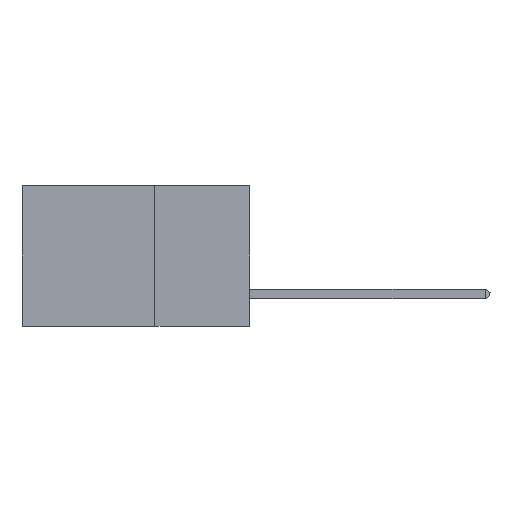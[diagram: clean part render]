
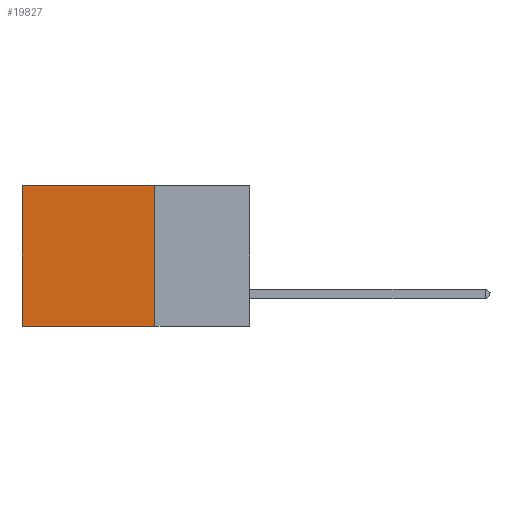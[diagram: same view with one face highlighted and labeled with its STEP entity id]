
A CAD part, left-side view. The second image highlights one B-rep face of the part: STEP entity #19827.
In plain terms, the highlighted planar face has unit normal (-1, 0, 0).
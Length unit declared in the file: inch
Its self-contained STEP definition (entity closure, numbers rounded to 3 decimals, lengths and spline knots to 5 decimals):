
#174 = EDGE_CURVE ( 'NONE', #9367, #7639, #6510, .T. ) ;
#503 = VERTEX_POINT ( 'NONE', #18927 ) ;
#1155 = ORIENTED_EDGE ( 'NONE', *, *, #21049, .F. ) ;
#1613 = CARTESIAN_POINT ( 'NONE',  ( 0.2875, 0.25, -0.37 ) ) ;
#5132 = ORIENTED_EDGE ( 'NONE', *, *, #18564, .T. ) ;
#6510 = LINE ( 'NONE', #1613, #17146 ) ;
#7128 = VECTOR ( 'NONE', #24020, 39.37008 ) ;
#7312 = DIRECTION ( 'NONE',  ( 0., 1., 0. ) ) ;
#7639 = VERTEX_POINT ( 'NONE', #15843 ) ;
#7976 = LINE ( 'NONE', #23427, #15790 ) ;
#9364 = AXIS2_PLACEMENT_3D ( 'NONE', #12331, #18625, #16492 ) ;
#9367 = VERTEX_POINT ( 'NONE', #23784 ) ;
#11425 = EDGE_LOOP ( 'NONE', ( #5132, #20590, #1155, #17836 ) ) ;
#11676 = DIRECTION ( 'NONE',  ( 0., 1., 0. ) ) ;
#11764 = EDGE_CURVE ( 'NONE', #503, #22747, #7976, .T. ) ;
#11805 = CARTESIAN_POINT ( 'NONE',  ( 0.2875, 0.25, 0. ) ) ;
#12331 = CARTESIAN_POINT ( 'NONE',  ( 0.2875, 0.25, 0. ) ) ;
#12833 = LINE ( 'NONE', #13109, #12863 ) ;
#12863 = VECTOR ( 'NONE', #19253, 39.37008 ) ;
#13109 = CARTESIAN_POINT ( 'NONE',  ( 0.2875, 0.6, 0. ) ) ;
#15790 = VECTOR ( 'NONE', #7312, 39.37008 ) ;
#15843 = CARTESIAN_POINT ( 'NONE',  ( 0.2875, 0.6, -0.37 ) ) ;
#16492 = DIRECTION ( 'NONE',  ( 0., 0., -1. ) ) ;
#17146 = VECTOR ( 'NONE', #11676, 39.37008 ) ;
#17836 = ORIENTED_EDGE ( 'NONE', *, *, #11764, .T. ) ;
#18387 = LINE ( 'NONE', #11805, #7128 ) ;
#18564 = EDGE_CURVE ( 'NONE', #22747, #7639, #12833, .T. ) ;
#18625 = DIRECTION ( 'NONE',  ( 1., 0., 0. ) ) ;
#18927 = CARTESIAN_POINT ( 'NONE',  ( 0.2875, 0.25, 0. ) ) ;
#19253 = DIRECTION ( 'NONE',  ( 0., 0., -1. ) ) ;
#19827 = ADVANCED_FACE ( 'NONE', ( #22830 ), #20473, .F. ) ;
#20473 = PLANE ( 'NONE',  #9364 ) ;
#20590 = ORIENTED_EDGE ( 'NONE', *, *, #174, .F. ) ;
#21049 = EDGE_CURVE ( 'NONE', #503, #9367, #18387, .T. ) ;
#21514 = CARTESIAN_POINT ( 'NONE',  ( 0.2875, 0.6, 0. ) ) ;
#22747 = VERTEX_POINT ( 'NONE', #21514 ) ;
#22830 = FACE_OUTER_BOUND ( 'NONE', #11425, .T. ) ;
#23427 = CARTESIAN_POINT ( 'NONE',  ( 0.2875, 0.25, 0. ) ) ;
#23784 = CARTESIAN_POINT ( 'NONE',  ( 0.2875, 0.25, -0.37 ) ) ;
#24020 = DIRECTION ( 'NONE',  ( 0., 0., -1. ) ) ;
